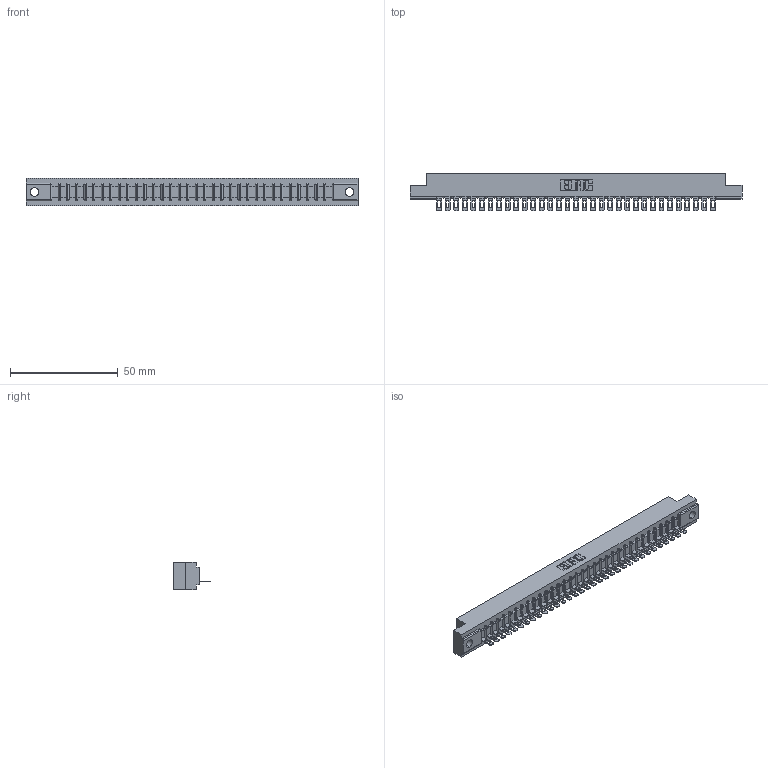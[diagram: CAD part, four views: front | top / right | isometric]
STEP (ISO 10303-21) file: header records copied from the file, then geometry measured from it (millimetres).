
FILE_DESCRIPTION (( 'STEP AP203' ), '1' );
FILE_NAME ('307-033-501-104.STEP', '2019-09-05T05:45:13', ( '' ), ( '' ), 'SwSTEP 2.0', 'SolidWorks 2016', '' );
FILE_SCHEMA (( 'CONFIG_CONTROL_DESIGN' ));
Length unit declared in the file: inch
Products named in the file (3): 307 Part_.156 Dia Mounting Holes; 307-033-501-104; 307-290-002_501
Assembly tree (34 placements, depth 2):
  307-033-501-104
    307 Part_.156 Dia Mounting Holes
    307-290-002_501  x33
Bounding box: 153.77 x 17.42 x 12.7 mm (x, y, z)
Volume: 16311.2 mm3; surface area: 20370.7 mm2
Topology: 34 solids, 34 shells, 2674 faces, 8213 edges, 5382 vertices
Faces by surface type: plane 1536, cylinder 1070, sphere 68
Entity records: 30612 total; most frequent: CARTESIAN_POINT 5166, ORIENTED_EDGE 5154, DIRECTION 5019, EDGE_CURVE 2577, LINE 1973, VECTOR 1973, VERTEX_POINT 1670, AXIS2_PLACEMENT_3D 1523
